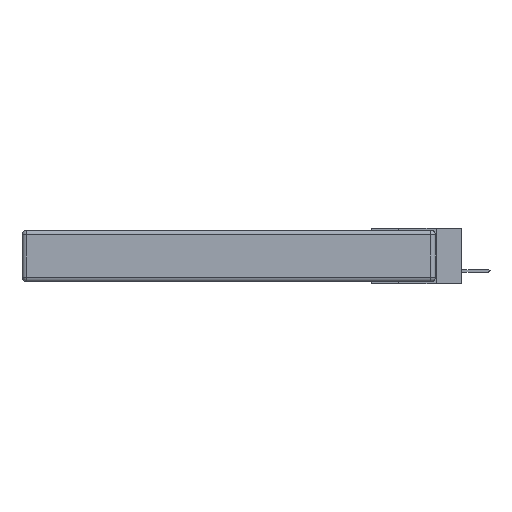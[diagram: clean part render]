
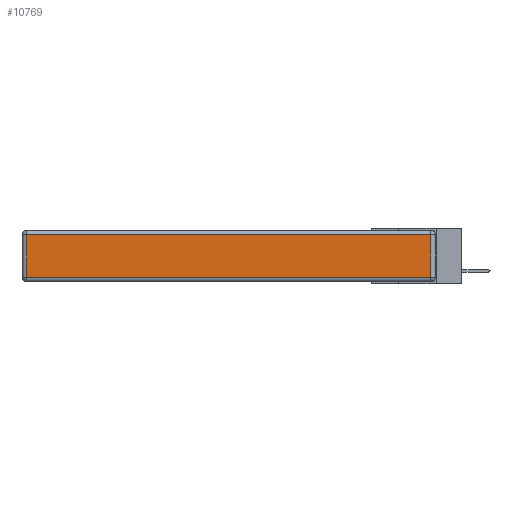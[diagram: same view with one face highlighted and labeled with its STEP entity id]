
A CAD part, left-side view. The second image highlights one B-rep face of the part: STEP entity #10769.
In plain terms, the highlighted planar face has unit normal (-1, 0, 0).
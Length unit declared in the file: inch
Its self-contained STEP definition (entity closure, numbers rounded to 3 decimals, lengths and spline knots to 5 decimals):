
#955 = VERTEX_POINT ( 'NONE', #14999 ) ;
#1594 = DIRECTION ( 'NONE',  ( 0., 0., 1. ) ) ;
#1881 = CARTESIAN_POINT ( 'NONE',  ( 0., 2.72, -0.343 ) ) ;
#2058 = AXIS2_PLACEMENT_3D ( 'NONE', #5033, #6265, #14817 ) ;
#2077 = FACE_OUTER_BOUND ( 'NONE', #15731, .T. ) ;
#4275 = ORIENTED_EDGE ( 'NONE', *, *, #9990, .T. ) ;
#4712 = VERTEX_POINT ( 'NONE', #13063 ) ;
#5033 = CARTESIAN_POINT ( 'NONE',  ( 0., 0., -0.343 ) ) ;
#5414 = EDGE_CURVE ( 'NONE', #955, #10491, #6893, .T. ) ;
#5969 = VERTEX_POINT ( 'NONE', #12297 ) ;
#6265 = DIRECTION ( 'NONE',  ( -1., 0., 0. ) ) ;
#6893 = LINE ( 'NONE', #8076, #7840 ) ;
#7130 = VECTOR ( 'NONE', #1594, 39.37008 ) ;
#7840 = VECTOR ( 'NONE', #9082, 39.37008 ) ;
#8076 = CARTESIAN_POINT ( 'NONE',  ( 0., 2.75, -0.03 ) ) ;
#8275 = LINE ( 'NONE', #1881, #15741 ) ;
#8463 = CARTESIAN_POINT ( 'NONE',  ( 0., 0.03, -0.343 ) ) ;
#9082 = DIRECTION ( 'NONE',  ( 0., 1., 0. ) ) ;
#9990 = EDGE_CURVE ( 'NONE', #4712, #5969, #10991, .T. ) ;
#10336 = LINE ( 'NONE', #8463, #7130 ) ;
#10491 = VERTEX_POINT ( 'NONE', #15368 ) ;
#10769 = ADVANCED_FACE ( 'NONE', ( #2077 ), #13353, .T. ) ;
#10991 = LINE ( 'NONE', #14410, #12717 ) ;
#11987 = DIRECTION ( 'NONE',  ( 0., -1., 0. ) ) ;
#12297 = CARTESIAN_POINT ( 'NONE',  ( 0., 0.03, -0.313 ) ) ;
#12517 = EDGE_CURVE ( 'NONE', #10491, #4712, #8275, .T. ) ;
#12717 = VECTOR ( 'NONE', #11987, 39.37008 ) ;
#12921 = DIRECTION ( 'NONE',  ( 0., 0., -1. ) ) ;
#13063 = CARTESIAN_POINT ( 'NONE',  ( 0., 2.72, -0.313 ) ) ;
#13078 = EDGE_CURVE ( 'NONE', #5969, #955, #10336, .T. ) ;
#13353 = PLANE ( 'NONE',  #2058 ) ;
#14410 = CARTESIAN_POINT ( 'NONE',  ( 0., 0., -0.313 ) ) ;
#14817 = DIRECTION ( 'NONE',  ( 0., 0., 1. ) ) ;
#14999 = CARTESIAN_POINT ( 'NONE',  ( 0., 0.03, -0.03 ) ) ;
#15310 = ORIENTED_EDGE ( 'NONE', *, *, #12517, .T. ) ;
#15368 = CARTESIAN_POINT ( 'NONE',  ( 0., 2.72, -0.03 ) ) ;
#15395 = ORIENTED_EDGE ( 'NONE', *, *, #5414, .T. ) ;
#15525 = ORIENTED_EDGE ( 'NONE', *, *, #13078, .T. ) ;
#15731 = EDGE_LOOP ( 'NONE', ( #4275, #15525, #15395, #15310 ) ) ;
#15741 = VECTOR ( 'NONE', #12921, 39.37008 ) ;
